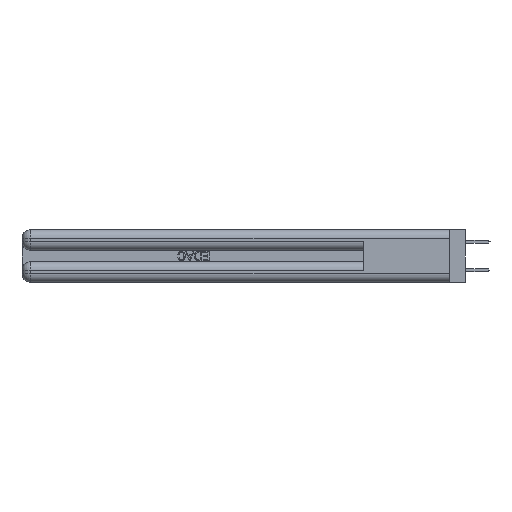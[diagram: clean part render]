
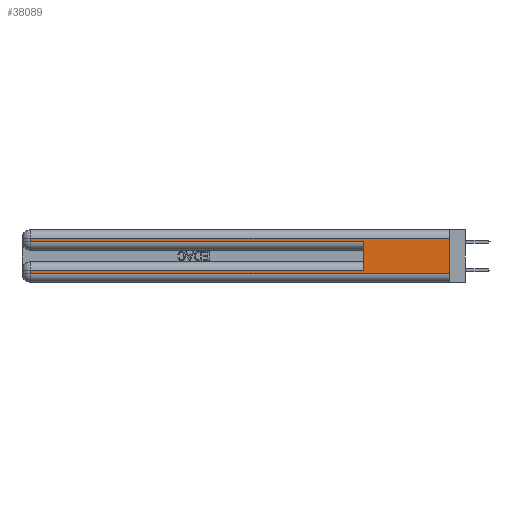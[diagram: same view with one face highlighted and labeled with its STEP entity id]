
A CAD part, left-side view. The second image highlights one B-rep face of the part: STEP entity #38089.
In plain terms, the highlighted planar face has unit normal (-1, 0, 0).
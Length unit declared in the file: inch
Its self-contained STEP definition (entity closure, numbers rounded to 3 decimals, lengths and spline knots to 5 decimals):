
#50 = LINE ( 'NONE', #25513, #34315 ) ;
#1378 = ORIENTED_EDGE ( 'NONE', *, *, #25821, .T. ) ;
#1632 = CARTESIAN_POINT ( 'NONE',  ( 0., 2.94, 0.285 ) ) ;
#2709 = DIRECTION ( 'NONE',  ( 0., -1., 0. ) ) ;
#2800 = EDGE_CURVE ( 'NONE', #3773, #23753, #19419, .T. ) ;
#3420 = VERTEX_POINT ( 'NONE', #1632 ) ;
#3773 = VERTEX_POINT ( 'NONE', #37959 ) ;
#4082 = EDGE_CURVE ( 'NONE', #26831, #23753, #50, .T. ) ;
#4281 = ORIENTED_EDGE ( 'NONE', *, *, #31512, .T. ) ;
#5686 = VECTOR ( 'NONE', #10385, 39.37008 ) ;
#7395 = LINE ( 'NONE', #28031, #8956 ) ;
#7525 = VERTEX_POINT ( 'NONE', #7813 ) ;
#7813 = CARTESIAN_POINT ( 'NONE',  ( 0., 0.6, 0.085 ) ) ;
#7979 = CARTESIAN_POINT ( 'NONE',  ( 0., 0., 0.31 ) ) ;
#8388 = EDGE_CURVE ( 'NONE', #7525, #33158, #7395, .T. ) ;
#8390 = CARTESIAN_POINT ( 'NONE',  ( 0., 2.94, 0.085 ) ) ;
#8811 = DIRECTION ( 'NONE',  ( 0., 0., -1. ) ) ;
#8956 = VECTOR ( 'NONE', #17870, 39.37008 ) ;
#9353 = CARTESIAN_POINT ( 'NONE',  ( 0., 0., 0.06 ) ) ;
#9773 = ORIENTED_EDGE ( 'NONE', *, *, #2800, .T. ) ;
#9867 = CARTESIAN_POINT ( 'NONE',  ( 0., 0., 0.31 ) ) ;
#10152 = ORIENTED_EDGE ( 'NONE', *, *, #32775, .T. ) ;
#10385 = DIRECTION ( 'NONE',  ( 0., 0., -1. ) ) ;
#11675 = DIRECTION ( 'NONE',  ( 0., 0., -1. ) ) ;
#11943 = VERTEX_POINT ( 'NONE', #8390 ) ;
#12164 = ORIENTED_EDGE ( 'NONE', *, *, #4082, .F. ) ;
#12882 = DIRECTION ( 'NONE',  ( 0., 1., 0. ) ) ;
#13908 = CARTESIAN_POINT ( 'NONE',  ( 0., 2.94, 0.37 ) ) ;
#14155 = EDGE_CURVE ( 'NONE', #24482, #3420, #26818, .T. ) ;
#16625 = EDGE_CURVE ( 'NONE', #7525, #11943, #30721, .T. ) ;
#17870 = DIRECTION ( 'NONE',  ( 0., 0., 1. ) ) ;
#18103 = CARTESIAN_POINT ( 'NONE',  ( 0., 0., 0.37 ) ) ;
#19419 = LINE ( 'NONE', #32316, #30297 ) ;
#20576 = VECTOR ( 'NONE', #28604, 39.37008 ) ;
#21426 = VECTOR ( 'NONE', #28907, 39.37008 ) ;
#21584 = DIRECTION ( 'NONE',  ( 1., 0., 0. ) ) ;
#23753 = VERTEX_POINT ( 'NONE', #9353 ) ;
#24085 = DIRECTION ( 'NONE',  ( 0., -1., 0. ) ) ;
#24241 = VECTOR ( 'NONE', #12882, 39.37008 ) ;
#24482 = VERTEX_POINT ( 'NONE', #27350 ) ;
#24725 = EDGE_LOOP ( 'NONE', ( #12164, #1378, #41674, #4281, #37245, #34129, #10152, #9773 ) ) ;
#25216 = CARTESIAN_POINT ( 'NONE',  ( 0., 0.6, 0.285 ) ) ;
#25513 = CARTESIAN_POINT ( 'NONE',  ( 0., 0., 0.37 ) ) ;
#25821 = EDGE_CURVE ( 'NONE', #26831, #24482, #32023, .T. ) ;
#26818 = LINE ( 'NONE', #13908, #20576 ) ;
#26831 = VERTEX_POINT ( 'NONE', #7979 ) ;
#27350 = CARTESIAN_POINT ( 'NONE',  ( 0., 2.94, 0.31 ) ) ;
#28031 = CARTESIAN_POINT ( 'NONE',  ( 0., 0.6, 0.145 ) ) ;
#28129 = LINE ( 'NONE', #33606, #32294 ) ;
#28604 = DIRECTION ( 'NONE',  ( 0., 0., -1. ) ) ;
#28907 = DIRECTION ( 'NONE',  ( 0., 1., 0. ) ) ;
#30297 = VECTOR ( 'NONE', #2709, 39.37008 ) ;
#30721 = LINE ( 'NONE', #31522, #21426 ) ;
#31504 = AXIS2_PLACEMENT_3D ( 'NONE', #18103, #21584, #11675 ) ;
#31512 = EDGE_CURVE ( 'NONE', #3420, #33158, #28129, .T. ) ;
#31522 = CARTESIAN_POINT ( 'NONE',  ( 0., 0., 0.085 ) ) ;
#32023 = LINE ( 'NONE', #9867, #24241 ) ;
#32175 = LINE ( 'NONE', #39568, #5686 ) ;
#32294 = VECTOR ( 'NONE', #24085, 39.37008 ) ;
#32316 = CARTESIAN_POINT ( 'NONE',  ( 0., 0., 0.06 ) ) ;
#32775 = EDGE_CURVE ( 'NONE', #11943, #3773, #32175, .T. ) ;
#33158 = VERTEX_POINT ( 'NONE', #25216 ) ;
#33606 = CARTESIAN_POINT ( 'NONE',  ( 0., 0., 0.285 ) ) ;
#34129 = ORIENTED_EDGE ( 'NONE', *, *, #16625, .T. ) ;
#34315 = VECTOR ( 'NONE', #8811, 39.37008 ) ;
#37245 = ORIENTED_EDGE ( 'NONE', *, *, #8388, .F. ) ;
#37959 = CARTESIAN_POINT ( 'NONE',  ( 0., 2.94, 0.06 ) ) ;
#38058 = PLANE ( 'NONE',  #31504 ) ;
#38089 = ADVANCED_FACE ( 'NONE', ( #42038 ), #38058, .F. ) ;
#39568 = CARTESIAN_POINT ( 'NONE',  ( 0., 2.94, 0.37 ) ) ;
#41674 = ORIENTED_EDGE ( 'NONE', *, *, #14155, .T. ) ;
#42038 = FACE_OUTER_BOUND ( 'NONE', #24725, .T. ) ;
